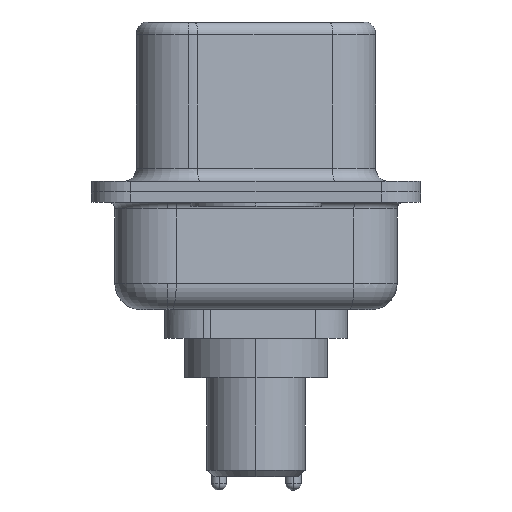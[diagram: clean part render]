
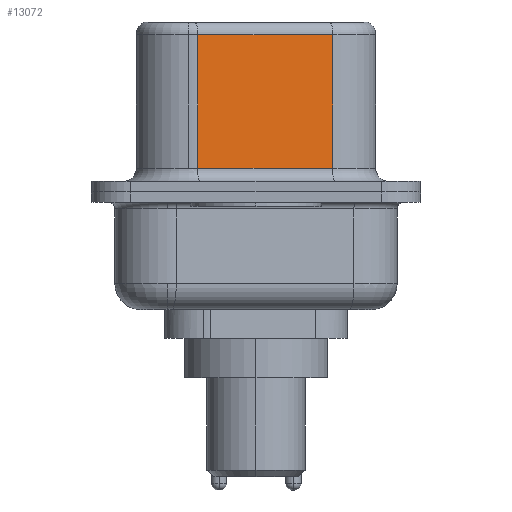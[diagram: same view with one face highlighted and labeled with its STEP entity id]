
A CAD part, left-side view. The second image highlights one B-rep face of the part: STEP entity #13072.
In plain terms, the highlighted planar face has unit normal (-0.985, -0.174, 0).
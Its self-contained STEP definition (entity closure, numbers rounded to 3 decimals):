
#1315 = CARTESIAN_POINT ( 'NONE',  ( 4.585, -2.927, 6.52 ) ) ;
#1824 = LINE ( 'NONE', #10834, #5209 ) ;
#2016 = CARTESIAN_POINT ( 'NONE',  ( 4.585, -2.927, 6.02 ) ) ;
#2221 = VECTOR ( 'NONE', #13221, 1000. ) ;
#2522 = DIRECTION ( 'NONE',  ( 0.174, -0.985, 0. ) ) ;
#2671 = DIRECTION ( 'NONE',  ( 0.985, 0.174, 0. ) ) ;
#3002 = FACE_OUTER_BOUND ( 'NONE', #8597, .T. ) ;
#3383 = CARTESIAN_POINT ( 'NONE',  ( 3.675, 2.233, 0.9 ) ) ;
#3500 = LINE ( 'NONE', #4151, #9834 ) ;
#3788 = EDGE_CURVE ( 'NONE', #14813, #6208, #3500, .T. ) ;
#3794 = ORIENTED_EDGE ( 'NONE', *, *, #6625, .T. ) ;
#4151 = CARTESIAN_POINT ( 'NONE',  ( 3.675, 2.233, 6.52 ) ) ;
#5209 = VECTOR ( 'NONE', #2522, 1000. ) ;
#5855 = DIRECTION ( 'NONE',  ( 0., 0., -1. ) ) ;
#6208 = VERTEX_POINT ( 'NONE', #3383 ) ;
#6332 = LINE ( 'NONE', #13023, #16052 ) ;
#6578 = EDGE_CURVE ( 'NONE', #9787, #14813, #15310, .T. ) ;
#6625 = EDGE_CURVE ( 'NONE', #6208, #15042, #1824, .T. ) ;
#7077 = CARTESIAN_POINT ( 'NONE',  ( 3.675, 2.233, 6.02 ) ) ;
#7514 = CARTESIAN_POINT ( 'NONE',  ( 4.585, -2.927, 0.9 ) ) ;
#8597 = EDGE_LOOP ( 'NONE', ( #12632, #14320, #14406, #3794 ) ) ;
#8768 = AXIS2_PLACEMENT_3D ( 'NONE', #1315, #2671, #11504 ) ;
#8991 = PLANE ( 'NONE',  #8768 ) ;
#9787 = VERTEX_POINT ( 'NONE', #2016 ) ;
#9834 = VECTOR ( 'NONE', #5855, 1000. ) ;
#10469 = DIRECTION ( 'NONE',  ( 0., 0., -1. ) ) ;
#10834 = CARTESIAN_POINT ( 'NONE',  ( 4.585, -2.927, 0.9 ) ) ;
#11504 = DIRECTION ( 'NONE',  ( -0.174, 0.985, 0. ) ) ;
#12359 = CARTESIAN_POINT ( 'NONE',  ( 4.585, -2.927, 6.02 ) ) ;
#12632 = ORIENTED_EDGE ( 'NONE', *, *, #14606, .F. ) ;
#13023 = CARTESIAN_POINT ( 'NONE',  ( 4.585, -2.927, 6.52 ) ) ;
#13072 = ADVANCED_FACE ( 'NONE', ( #3002 ), #8991, .F. ) ;
#13221 = DIRECTION ( 'NONE',  ( -0.174, 0.985, 0. ) ) ;
#14320 = ORIENTED_EDGE ( 'NONE', *, *, #6578, .T. ) ;
#14406 = ORIENTED_EDGE ( 'NONE', *, *, #3788, .T. ) ;
#14606 = EDGE_CURVE ( 'NONE', #9787, #15042, #6332, .T. ) ;
#14813 = VERTEX_POINT ( 'NONE', #7077 ) ;
#15042 = VERTEX_POINT ( 'NONE', #7514 ) ;
#15310 = LINE ( 'NONE', #12359, #2221 ) ;
#16052 = VECTOR ( 'NONE', #10469, 1000. ) ;
